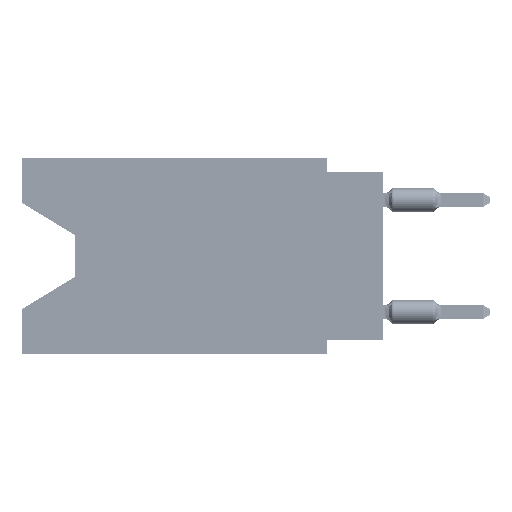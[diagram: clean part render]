
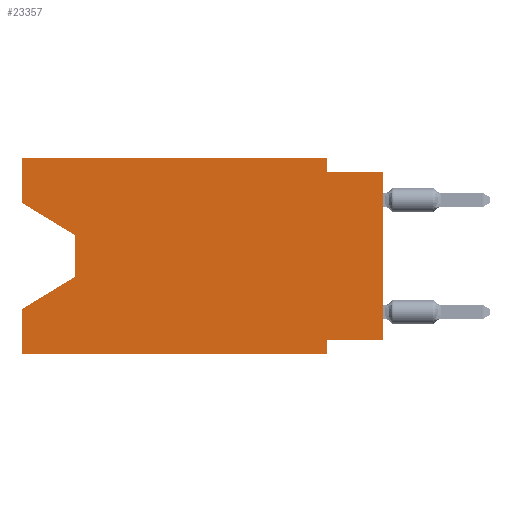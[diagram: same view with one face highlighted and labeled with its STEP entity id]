
A CAD part, left-side view. The second image highlights one B-rep face of the part: STEP entity #23357.
In plain terms, the highlighted planar face has unit normal (-1, 0, 0).
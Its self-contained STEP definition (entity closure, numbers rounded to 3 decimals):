
#166 = VERTEX_POINT ( 'NONE', #40773 ) ;
#307 = VECTOR ( 'NONE', #70680, 1000. ) ;
#386 = DIRECTION ( 'NONE',  ( 0., 1., 0. ) ) ;
#1797 = ORIENTED_EDGE ( 'NONE', *, *, #44656, .F. ) ;
#2812 = LINE ( 'NONE', #21109, #60732 ) ;
#8655 = CARTESIAN_POINT ( 'NONE',  ( 0., 2.54, -0.635 ) ) ;
#8862 = DIRECTION ( 'NONE',  ( 0., 0., 1. ) ) ;
#10156 = VECTOR ( 'NONE', #54092, 1000. ) ;
#10545 = VERTEX_POINT ( 'NONE', #19649 ) ;
#10894 = ORIENTED_EDGE ( 'NONE', *, *, #14882, .T. ) ;
#11356 = CARTESIAN_POINT ( 'NONE',  ( 0., 2.54, -8.89 ) ) ;
#12655 = EDGE_CURVE ( 'NONE', #34831, #46711, #40947, .T. ) ;
#13291 = EDGE_CURVE ( 'NONE', #20358, #30609, #25240, .T. ) ;
#13694 = AXIS2_PLACEMENT_3D ( 'NONE', #67102, #37525, #61267 ) ;
#14138 = EDGE_CURVE ( 'NONE', #44294, #34974, #29598, .T. ) ;
#14882 = EDGE_CURVE ( 'NONE', #66560, #166, #46582, .T. ) ;
#15316 = LINE ( 'NONE', #74067, #53666 ) ;
#16386 = VECTOR ( 'NONE', #35091, 1000. ) ;
#16849 = EDGE_CURVE ( 'NONE', #166, #68884, #25812, .T. ) ;
#17348 = VECTOR ( 'NONE', #386, 1000. ) ;
#19178 = CARTESIAN_POINT ( 'NONE',  ( 0., 13.97, -5.385 ) ) ;
#19643 = FACE_OUTER_BOUND ( 'NONE', #47042, .T. ) ;
#19649 = CARTESIAN_POINT ( 'NONE',  ( 0., 0., -8.255 ) ) ;
#20358 = VERTEX_POINT ( 'NONE', #43314 ) ;
#21109 = CARTESIAN_POINT ( 'NONE',  ( 0., 13.97, -5.385 ) ) ;
#21190 = VECTOR ( 'NONE', #27807, 1000. ) ;
#22781 = EDGE_CURVE ( 'NONE', #10545, #34831, #40513, .T. ) ;
#23357 = ADVANCED_FACE ( 'NONE', ( #19643 ), #43388, .F. ) ;
#25240 = LINE ( 'NONE', #66864, #58594 ) ;
#25812 = LINE ( 'NONE', #62368, #28066 ) ;
#27807 = DIRECTION ( 'NONE',  ( 0., 0., 1. ) ) ;
#28011 = CARTESIAN_POINT ( 'NONE',  ( 0., 0., 0. ) ) ;
#28066 = VECTOR ( 'NONE', #37867, 1000. ) ;
#28832 = CARTESIAN_POINT ( 'NONE',  ( 0., 0., -8.255 ) ) ;
#29598 = LINE ( 'NONE', #52956, #10156 ) ;
#30609 = VERTEX_POINT ( 'NONE', #38291 ) ;
#31178 = ORIENTED_EDGE ( 'NONE', *, *, #55821, .T. ) ;
#33573 = ORIENTED_EDGE ( 'NONE', *, *, #49215, .F. ) ;
#34831 = VERTEX_POINT ( 'NONE', #46570 ) ;
#34974 = VERTEX_POINT ( 'NONE', #74470 ) ;
#35091 = DIRECTION ( 'NONE',  ( 0., 0., -1. ) ) ;
#36621 = VERTEX_POINT ( 'NONE', #8655 ) ;
#37195 = EDGE_CURVE ( 'NONE', #10545, #75811, #71168, .T. ) ;
#37525 = DIRECTION ( 'NONE',  ( 1., 0., 0. ) ) ;
#37867 = DIRECTION ( 'NONE',  ( 0., 0., -1. ) ) ;
#38291 = CARTESIAN_POINT ( 'NONE',  ( 0., 16.383, -6.852 ) ) ;
#40513 = LINE ( 'NONE', #28832, #17348 ) ;
#40773 = CARTESIAN_POINT ( 'NONE',  ( 0., 13.97, -3.505 ) ) ;
#40947 = LINE ( 'NONE', #11356, #16386 ) ;
#41120 = CARTESIAN_POINT ( 'NONE',  ( 0., 16.383, 0. ) ) ;
#42965 = EDGE_CURVE ( 'NONE', #36621, #75811, #69115, .T. ) ;
#43314 = CARTESIAN_POINT ( 'NONE',  ( 0., 16.383, -8.89 ) ) ;
#43388 = PLANE ( 'NONE',  #13694 ) ;
#44294 = VERTEX_POINT ( 'NONE', #41120 ) ;
#44656 = EDGE_CURVE ( 'NONE', #66560, #44294, #51541, .T. ) ;
#45438 = ORIENTED_EDGE ( 'NONE', *, *, #50459, .T. ) ;
#45664 = ORIENTED_EDGE ( 'NONE', *, *, #12655, .F. ) ;
#45842 = ORIENTED_EDGE ( 'NONE', *, *, #13291, .F. ) ;
#46262 = CARTESIAN_POINT ( 'NONE',  ( 0., 16.383, -2.038 ) ) ;
#46570 = CARTESIAN_POINT ( 'NONE',  ( 0., 2.54, -8.255 ) ) ;
#46582 = LINE ( 'NONE', #69913, #307 ) ;
#46711 = VERTEX_POINT ( 'NONE', #55757 ) ;
#47042 = EDGE_LOOP ( 'NONE', ( #10894, #55865, #45438, #45842, #31178, #45664, #62230, #48634, #72869, #33573, #53455, #1797 ) ) ;
#47982 = DIRECTION ( 'NONE',  ( 0., -1., 0. ) ) ;
#48369 = VECTOR ( 'NONE', #47982, 1000. ) ;
#48634 = ORIENTED_EDGE ( 'NONE', *, *, #37195, .T. ) ;
#49215 = EDGE_CURVE ( 'NONE', #34974, #36621, #73777, .T. ) ;
#50274 = VECTOR ( 'NONE', #62102, 1000. ) ;
#50459 = EDGE_CURVE ( 'NONE', #68884, #30609, #2812, .T. ) ;
#51541 = LINE ( 'NONE', #51924, #21190 ) ;
#51589 = CARTESIAN_POINT ( 'NONE',  ( 0., 2.54, 0. ) ) ;
#51924 = CARTESIAN_POINT ( 'NONE',  ( 0., 16.383, 0. ) ) ;
#52956 = CARTESIAN_POINT ( 'NONE',  ( 0., 16.383, 0. ) ) ;
#53455 = ORIENTED_EDGE ( 'NONE', *, *, #14138, .F. ) ;
#53666 = VECTOR ( 'NONE', #67852, 1000. ) ;
#54092 = DIRECTION ( 'NONE',  ( 0., -1., 0. ) ) ;
#55757 = CARTESIAN_POINT ( 'NONE',  ( 0., 2.54, -8.89 ) ) ;
#55821 = EDGE_CURVE ( 'NONE', #20358, #46711, #15316, .T. ) ;
#55865 = ORIENTED_EDGE ( 'NONE', *, *, #16849, .T. ) ;
#56134 = DIRECTION ( 'NONE',  ( 0., 0.855, -0.519 ) ) ;
#58594 = VECTOR ( 'NONE', #8862, 1000. ) ;
#59269 = CARTESIAN_POINT ( 'NONE',  ( 0., 0., -0.635 ) ) ;
#60732 = VECTOR ( 'NONE', #56134, 1000. ) ;
#61267 = DIRECTION ( 'NONE',  ( 0., 0., -1. ) ) ;
#62102 = DIRECTION ( 'NONE',  ( 0., 0., -1. ) ) ;
#62230 = ORIENTED_EDGE ( 'NONE', *, *, #22781, .F. ) ;
#62368 = CARTESIAN_POINT ( 'NONE',  ( 0., 13.97, -3.505 ) ) ;
#63416 = DIRECTION ( 'NONE',  ( 0., 0., 1. ) ) ;
#66560 = VERTEX_POINT ( 'NONE', #46262 ) ;
#66864 = CARTESIAN_POINT ( 'NONE',  ( 0., 16.383, 0. ) ) ;
#67102 = CARTESIAN_POINT ( 'NONE',  ( 0., 16.383, 0. ) ) ;
#67620 = CARTESIAN_POINT ( 'NONE',  ( 0., 0., -0.635 ) ) ;
#67852 = DIRECTION ( 'NONE',  ( 0., -1., 0. ) ) ;
#68884 = VERTEX_POINT ( 'NONE', #19178 ) ;
#69115 = LINE ( 'NONE', #59269, #48369 ) ;
#69913 = CARTESIAN_POINT ( 'NONE',  ( 0., 16.383, -2.038 ) ) ;
#70680 = DIRECTION ( 'NONE',  ( 0., -0.855, -0.519 ) ) ;
#71168 = LINE ( 'NONE', #28011, #75235 ) ;
#72869 = ORIENTED_EDGE ( 'NONE', *, *, #42965, .F. ) ;
#73777 = LINE ( 'NONE', #51589, #50274 ) ;
#74067 = CARTESIAN_POINT ( 'NONE',  ( 0., 16.383, -8.89 ) ) ;
#74470 = CARTESIAN_POINT ( 'NONE',  ( 0., 2.54, 0. ) ) ;
#75235 = VECTOR ( 'NONE', #63416, 1000. ) ;
#75811 = VERTEX_POINT ( 'NONE', #67620 ) ;
